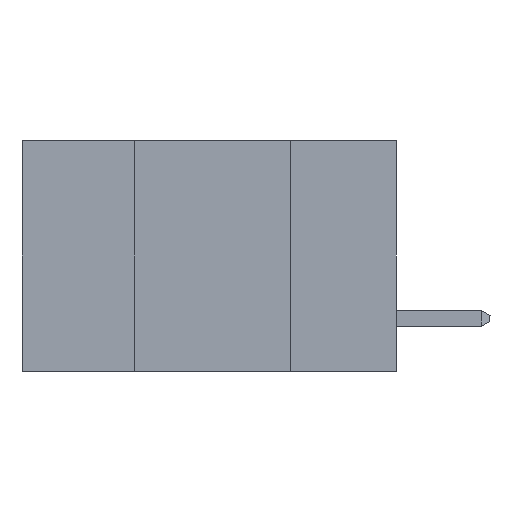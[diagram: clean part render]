
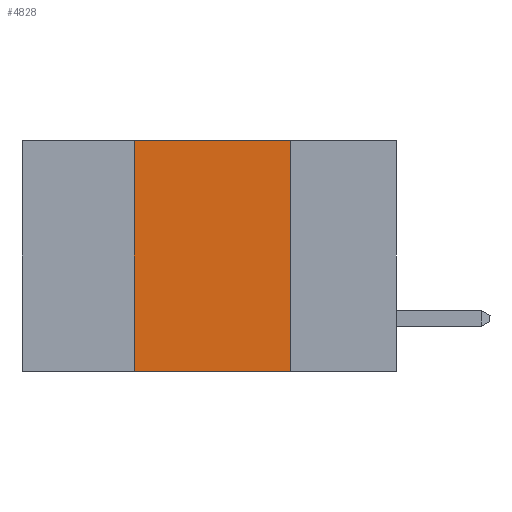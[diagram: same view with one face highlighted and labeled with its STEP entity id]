
A CAD part, left-side view. The second image highlights one B-rep face of the part: STEP entity #4828.
In plain terms, the highlighted planar face has unit normal (-1, 0, 0).
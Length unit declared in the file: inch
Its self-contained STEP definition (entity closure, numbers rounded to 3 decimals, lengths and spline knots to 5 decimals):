
#1216 = VERTEX_POINT ( 'NONE', #16462 ) ;
#1632 = LINE ( 'NONE', #4689, #12463 ) ;
#2030 = CARTESIAN_POINT ( 'NONE',  ( 0., 0.42, 0. ) ) ;
#2464 = FACE_OUTER_BOUND ( 'NONE', #13444, .T. ) ;
#3586 = CARTESIAN_POINT ( 'NONE',  ( 0., 0.42, -0.37 ) ) ;
#4122 = EDGE_CURVE ( 'NONE', #17395, #4733, #9816, .T. ) ;
#4404 = VECTOR ( 'NONE', #17559, 39.37008 ) ;
#4689 = CARTESIAN_POINT ( 'NONE',  ( 0., 0.17, -0.37 ) ) ;
#4733 = VERTEX_POINT ( 'NONE', #2030 ) ;
#4828 = ADVANCED_FACE ( 'NONE', ( #2464 ), #17691, .F. ) ;
#4830 = LINE ( 'NONE', #10592, #4404 ) ;
#6646 = DIRECTION ( 'NONE',  ( 0., 0., -1. ) ) ;
#7878 = EDGE_CURVE ( 'NONE', #17395, #1216, #16862, .T. ) ;
#8031 = AXIS2_PLACEMENT_3D ( 'NONE', #12200, #15024, #6646 ) ;
#8557 = ORIENTED_EDGE ( 'NONE', *, *, #7878, .T. ) ;
#9377 = VECTOR ( 'NONE', #12088, 39.37008 ) ;
#9391 = ORIENTED_EDGE ( 'NONE', *, *, #11195, .F. ) ;
#9816 = LINE ( 'NONE', #3586, #9377 ) ;
#10592 = CARTESIAN_POINT ( 'NONE',  ( 0., 0.6, 0. ) ) ;
#11195 = EDGE_CURVE ( 'NONE', #4733, #14424, #4830, .T. ) ;
#11459 = CARTESIAN_POINT ( 'NONE',  ( 0., 0.17, 0. ) ) ;
#11730 = ORIENTED_EDGE ( 'NONE', *, *, #4122, .F. ) ;
#12088 = DIRECTION ( 'NONE',  ( 0., 0., 1. ) ) ;
#12200 = CARTESIAN_POINT ( 'NONE',  ( 0., 0.6, 0. ) ) ;
#12244 = CARTESIAN_POINT ( 'NONE',  ( 0., 0.6, -0.37 ) ) ;
#12311 = DIRECTION ( 'NONE',  ( 0., -1., 0. ) ) ;
#12463 = VECTOR ( 'NONE', #15913, 39.37008 ) ;
#13444 = EDGE_LOOP ( 'NONE', ( #17418, #9391, #11730, #8557 ) ) ;
#14007 = EDGE_CURVE ( 'NONE', #14424, #1216, #1632, .T. ) ;
#14424 = VERTEX_POINT ( 'NONE', #11459 ) ;
#15024 = DIRECTION ( 'NONE',  ( 1., 0., 0. ) ) ;
#15913 = DIRECTION ( 'NONE',  ( 0., 0., -1. ) ) ;
#16415 = VECTOR ( 'NONE', #12311, 39.37008 ) ;
#16462 = CARTESIAN_POINT ( 'NONE',  ( 0., 0.17, -0.37 ) ) ;
#16862 = LINE ( 'NONE', #12244, #16415 ) ;
#17395 = VERTEX_POINT ( 'NONE', #17800 ) ;
#17418 = ORIENTED_EDGE ( 'NONE', *, *, #14007, .F. ) ;
#17559 = DIRECTION ( 'NONE',  ( 0., -1., 0. ) ) ;
#17691 = PLANE ( 'NONE',  #8031 ) ;
#17800 = CARTESIAN_POINT ( 'NONE',  ( 0., 0.42, -0.37 ) ) ;
